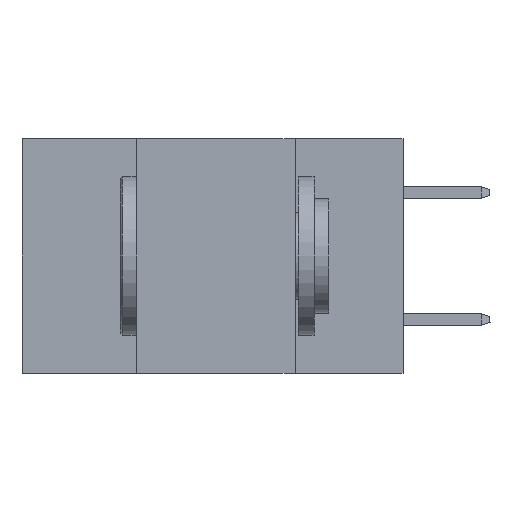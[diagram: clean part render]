
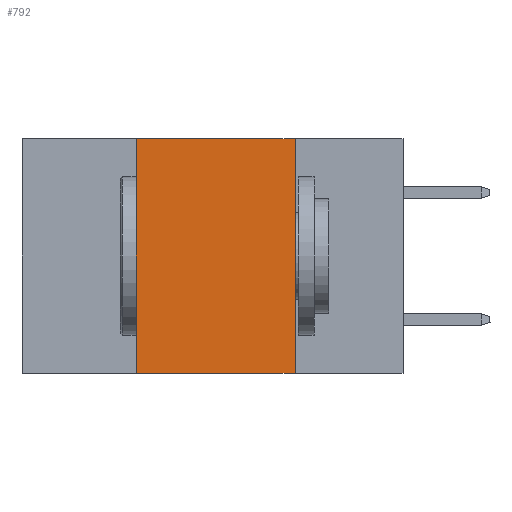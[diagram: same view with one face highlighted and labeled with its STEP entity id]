
A CAD part, left-side view. The second image highlights one B-rep face of the part: STEP entity #792.
In plain terms, the highlighted planar face has unit normal (-1, 0, 0).
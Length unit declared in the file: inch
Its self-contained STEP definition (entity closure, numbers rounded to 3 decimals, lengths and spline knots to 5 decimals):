
#119 = DIRECTION ( 'NONE',  ( 0., 0., -1. ) ) ;
#207 = PLANE ( 'NONE',  #2817 ) ;
#661 = LINE ( 'NONE', #11902, #4799 ) ;
#792 = ADVANCED_FACE ( 'NONE', ( #14335 ), #207, .F. ) ;
#2377 = CARTESIAN_POINT ( 'NONE',  ( 0., 0.17, -0.37 ) ) ;
#2381 = VECTOR ( 'NONE', #11218, 39.37008 ) ;
#2382 = EDGE_CURVE ( 'NONE', #9359, #14474, #661, .T. ) ;
#2561 = EDGE_CURVE ( 'NONE', #8444, #9359, #2870, .T. ) ;
#2587 = ORIENTED_EDGE ( 'NONE', *, *, #15122, .F. ) ;
#2817 = AXIS2_PLACEMENT_3D ( 'NONE', #3068, #4200, #119 ) ;
#2870 = LINE ( 'NONE', #7267, #17792 ) ;
#3068 = CARTESIAN_POINT ( 'NONE',  ( 0., 0.6, 0. ) ) ;
#3293 = ORIENTED_EDGE ( 'NONE', *, *, #2561, .F. ) ;
#4200 = DIRECTION ( 'NONE',  ( 1., 0., 0. ) ) ;
#4799 = VECTOR ( 'NONE', #14890, 39.37008 ) ;
#6705 = CARTESIAN_POINT ( 'NONE',  ( 0., 0.42, 0. ) ) ;
#6907 = EDGE_CURVE ( 'NONE', #15058, #14474, #17993, .T. ) ;
#7267 = CARTESIAN_POINT ( 'NONE',  ( 0., 0.6, 0. ) ) ;
#8444 = VERTEX_POINT ( 'NONE', #6705 ) ;
#9359 = VERTEX_POINT ( 'NONE', #10923 ) ;
#10798 = LINE ( 'NONE', #13681, #16303 ) ;
#10923 = CARTESIAN_POINT ( 'NONE',  ( 0., 0.17, 0. ) ) ;
#11218 = DIRECTION ( 'NONE',  ( 0., -1., 0. ) ) ;
#11902 = CARTESIAN_POINT ( 'NONE',  ( 0., 0.17, 0. ) ) ;
#12615 = CARTESIAN_POINT ( 'NONE',  ( 0., 0.6, -0.37 ) ) ;
#12633 = DIRECTION ( 'NONE',  ( 0., -1., 0. ) ) ;
#13580 = DIRECTION ( 'NONE',  ( 0., 0., 1. ) ) ;
#13681 = CARTESIAN_POINT ( 'NONE',  ( 0., 0.42, 0. ) ) ;
#14335 = FACE_OUTER_BOUND ( 'NONE', #17530, .T. ) ;
#14429 = ORIENTED_EDGE ( 'NONE', *, *, #6907, .T. ) ;
#14474 = VERTEX_POINT ( 'NONE', #2377 ) ;
#14514 = CARTESIAN_POINT ( 'NONE',  ( 0., 0.42, -0.37 ) ) ;
#14890 = DIRECTION ( 'NONE',  ( 0., 0., -1. ) ) ;
#15058 = VERTEX_POINT ( 'NONE', #14514 ) ;
#15122 = EDGE_CURVE ( 'NONE', #15058, #8444, #10798, .T. ) ;
#15366 = ORIENTED_EDGE ( 'NONE', *, *, #2382, .F. ) ;
#16303 = VECTOR ( 'NONE', #13580, 39.37008 ) ;
#17530 = EDGE_LOOP ( 'NONE', ( #15366, #3293, #2587, #14429 ) ) ;
#17792 = VECTOR ( 'NONE', #12633, 39.37008 ) ;
#17993 = LINE ( 'NONE', #12615, #2381 ) ;
